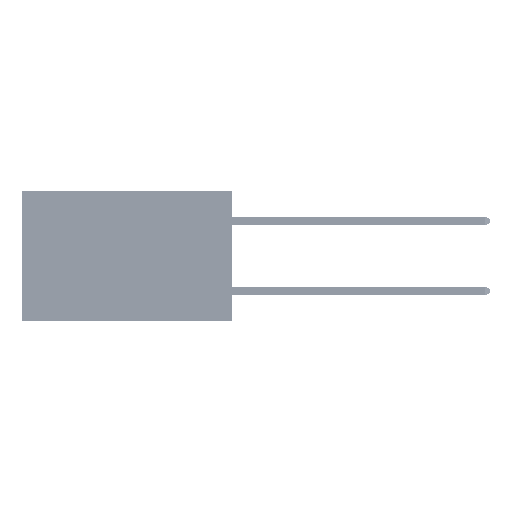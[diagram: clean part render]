
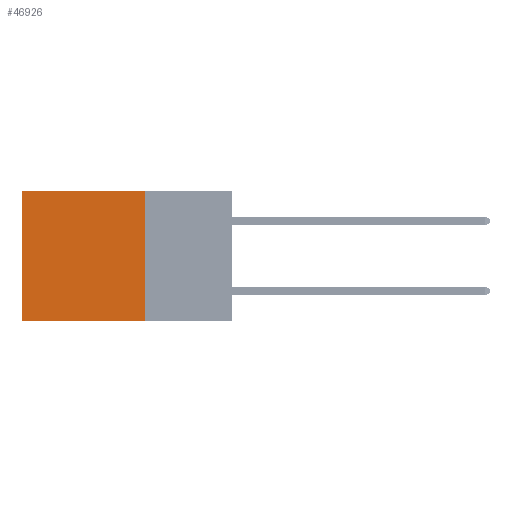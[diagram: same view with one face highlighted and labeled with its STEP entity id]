
A CAD part, left-side view. The second image highlights one B-rep face of the part: STEP entity #46926.
In plain terms, the highlighted planar face has unit normal (-1, 0, 0).
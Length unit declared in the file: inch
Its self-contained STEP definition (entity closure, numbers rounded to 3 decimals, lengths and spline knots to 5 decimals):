
#1056 = VECTOR ( 'NONE', #30599, 39.37008 ) ;
#1101 = DIRECTION ( 'NONE',  ( 0., 0., -1. ) ) ;
#1127 = VERTEX_POINT ( 'NONE', #16201 ) ;
#2478 = VERTEX_POINT ( 'NONE', #48324 ) ;
#2486 = EDGE_CURVE ( 'NONE', #13909, #1127, #20461, .T. ) ;
#2747 = ORIENTED_EDGE ( 'NONE', *, *, #40858, .T. ) ;
#4450 = CARTESIAN_POINT ( 'NONE',  ( 0.2875, 0.25, -0.37 ) ) ;
#10767 = DIRECTION ( 'NONE',  ( 0., 1., 0. ) ) ;
#10970 = ORIENTED_EDGE ( 'NONE', *, *, #14012, .T. ) ;
#11150 = ORIENTED_EDGE ( 'NONE', *, *, #44493, .F. ) ;
#13148 = CARTESIAN_POINT ( 'NONE',  ( 0.2875, 0.25, 0. ) ) ;
#13909 = VERTEX_POINT ( 'NONE', #13148 ) ;
#14012 = EDGE_CURVE ( 'NONE', #2478, #47889, #19258, .T. ) ;
#15242 = CARTESIAN_POINT ( 'NONE',  ( 0.2875, 0.25, 0. ) ) ;
#16201 = CARTESIAN_POINT ( 'NONE',  ( 0.2875, 0.25, -0.37 ) ) ;
#17799 = VECTOR ( 'NONE', #10767, 39.37008 ) ;
#19258 = LINE ( 'NONE', #46361, #1056 ) ;
#20461 = LINE ( 'NONE', #39829, #42373 ) ;
#20919 = ORIENTED_EDGE ( 'NONE', *, *, #2486, .F. ) ;
#22979 = DIRECTION ( 'NONE',  ( 1., 0., 0. ) ) ;
#26348 = EDGE_LOOP ( 'NONE', ( #10970, #11150, #20919, #2747 ) ) ;
#30599 = DIRECTION ( 'NONE',  ( 0., 0., -1. ) ) ;
#30953 = DIRECTION ( 'NONE',  ( 0., 0., -1. ) ) ;
#34832 = FACE_OUTER_BOUND ( 'NONE', #26348, .T. ) ;
#36413 = DIRECTION ( 'NONE',  ( 0., 1., 0. ) ) ;
#38657 = VECTOR ( 'NONE', #36413, 39.37008 ) ;
#39829 = CARTESIAN_POINT ( 'NONE',  ( 0.2875, 0.25, 0. ) ) ;
#40858 = EDGE_CURVE ( 'NONE', #13909, #2478, #50492, .T. ) ;
#41258 = AXIS2_PLACEMENT_3D ( 'NONE', #15242, #22979, #30953 ) ;
#41489 = CARTESIAN_POINT ( 'NONE',  ( 0.2875, 0.25, 0. ) ) ;
#42373 = VECTOR ( 'NONE', #1101, 39.37008 ) ;
#43342 = PLANE ( 'NONE',  #41258 ) ;
#43655 = LINE ( 'NONE', #4450, #38657 ) ;
#44493 = EDGE_CURVE ( 'NONE', #1127, #47889, #43655, .T. ) ;
#44679 = CARTESIAN_POINT ( 'NONE',  ( 0.2875, 0.6, -0.37 ) ) ;
#46361 = CARTESIAN_POINT ( 'NONE',  ( 0.2875, 0.6, 0. ) ) ;
#46926 = ADVANCED_FACE ( 'NONE', ( #34832 ), #43342, .F. ) ;
#47889 = VERTEX_POINT ( 'NONE', #44679 ) ;
#48324 = CARTESIAN_POINT ( 'NONE',  ( 0.2875, 0.6, 0. ) ) ;
#50492 = LINE ( 'NONE', #41489, #17799 ) ;
